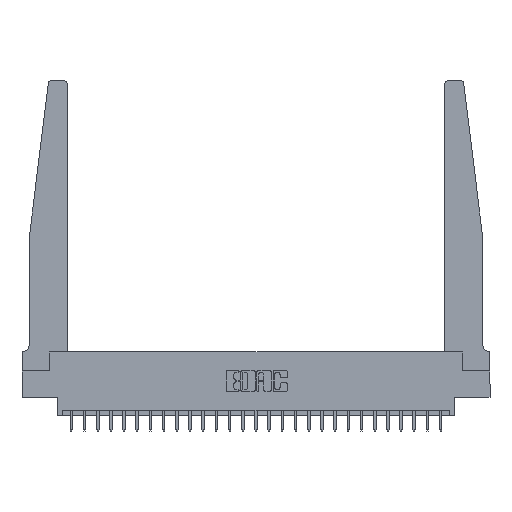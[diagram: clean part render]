
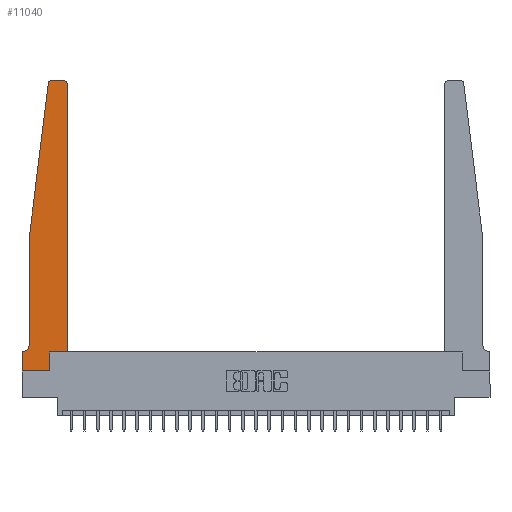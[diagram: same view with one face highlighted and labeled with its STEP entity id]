
A CAD part, top view. The second image highlights one B-rep face of the part: STEP entity #11040.
In plain terms, the highlighted planar face has unit normal (0, 0, 1).
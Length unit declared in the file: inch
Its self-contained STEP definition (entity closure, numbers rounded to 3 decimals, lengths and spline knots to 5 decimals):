
#15 = VECTOR ( 'NONE', #23621, 39.37008 ) ;
#415 = ORIENTED_EDGE ( 'NONE', *, *, #13755, .T. ) ;
#443 = CIRCLE ( 'NONE', #2517, 0.05 ) ;
#631 = CARTESIAN_POINT ( 'NONE',  ( 0.065, 0.1875, 0.37 ) ) ;
#632 = LINE ( 'NONE', #10656, #8835 ) ;
#813 = CARTESIAN_POINT ( 'NONE',  ( 0., 0., 0.37 ) ) ;
#1310 = CARTESIAN_POINT ( 'NONE',  ( 0.425, 0.18, 0.37 ) ) ;
#1545 = DIRECTION ( 'NONE',  ( 0., 0., 1. ) ) ;
#2093 = CARTESIAN_POINT ( 'NONE',  ( 0.395, 2.72, 0.37 ) ) ;
#2231 = LINE ( 'NONE', #12659, #4128 ) ;
#2368 = PLANE ( 'NONE',  #19766 ) ;
#2517 = AXIS2_PLACEMENT_3D ( 'NONE', #11095, #19156, #23111 ) ;
#2625 = ORIENTED_EDGE ( 'NONE', *, *, #9201, .T. ) ;
#3058 = VERTEX_POINT ( 'NONE', #9510 ) ;
#3242 = VECTOR ( 'NONE', #24822, 39.37008 ) ;
#3531 = LINE ( 'NONE', #3913, #18359 ) ;
#3632 = CARTESIAN_POINT ( 'NONE',  ( 0.065, 1.25, 0.37 ) ) ;
#3913 = CARTESIAN_POINT ( 'NONE',  ( 0.425, 0.18, 0.37 ) ) ;
#4128 = VECTOR ( 'NONE', #24389, 39.37008 ) ;
#5213 = ORIENTED_EDGE ( 'NONE', *, *, #22610, .T. ) ;
#5473 = VERTEX_POINT ( 'NONE', #18011 ) ;
#6308 = DIRECTION ( 'NONE',  ( 1., 0., 0. ) ) ;
#6482 = CARTESIAN_POINT ( 'NONE',  ( 0.24675, 2.72367, 0.37 ) ) ;
#6563 = LINE ( 'NONE', #631, #15560 ) ;
#6624 = EDGE_CURVE ( 'NONE', #25329, #9473, #9334, .T. ) ;
#6874 = ORIENTED_EDGE ( 'NONE', *, *, #20873, .T. ) ;
#6948 = VECTOR ( 'NONE', #25682, 39.37008 ) ;
#7537 = ORIENTED_EDGE ( 'NONE', *, *, #6624, .T. ) ;
#7592 = DIRECTION ( 'NONE',  ( 1., 0., 0. ) ) ;
#8638 = CARTESIAN_POINT ( 'NONE',  ( 0.065, 0.2375, 0.37 ) ) ;
#8674 = DIRECTION ( 'NONE',  ( -1., 0., 0. ) ) ;
#8703 = DIRECTION ( 'NONE',  ( 0., 0., 1. ) ) ;
#8835 = VECTOR ( 'NONE', #12514, 39.37008 ) ;
#9074 = VERTEX_POINT ( 'NONE', #6482 ) ;
#9201 = EDGE_CURVE ( 'NONE', #3058, #18370, #18778, .T. ) ;
#9250 = CARTESIAN_POINT ( 'NONE',  ( 0.27653, 2.75, 0.37 ) ) ;
#9334 = CIRCLE ( 'NONE', #19443, 0.03 ) ;
#9455 = CARTESIAN_POINT ( 'NONE',  ( 0.27653, 2.72, 0.37 ) ) ;
#9473 = VERTEX_POINT ( 'NONE', #9993 ) ;
#9510 = CARTESIAN_POINT ( 'NONE',  ( 0., 0., 0.37 ) ) ;
#9621 = DIRECTION ( 'NONE',  ( -1., 0., 0. ) ) ;
#9673 = EDGE_CURVE ( 'NONE', #19963, #3058, #2231, .T. ) ;
#9875 = LINE ( 'NONE', #19652, #23726 ) ;
#9993 = CARTESIAN_POINT ( 'NONE',  ( 0.395, 2.75, 0.37 ) ) ;
#10405 = DIRECTION ( 'NONE',  ( 0., 0., 1. ) ) ;
#10418 = DIRECTION ( 'NONE',  ( 1., 0., 0. ) ) ;
#10619 = CARTESIAN_POINT ( 'NONE',  ( 0.2605, 0.18, 0.37 ) ) ;
#10656 = CARTESIAN_POINT ( 'NONE',  ( 0.065, 1.25, 0.37 ) ) ;
#10702 = VERTEX_POINT ( 'NONE', #10619 ) ;
#10730 = CARTESIAN_POINT ( 'NONE',  ( 0.425, 0.18, 0.37 ) ) ;
#11040 = ADVANCED_FACE ( 'NONE', ( #20434 ), #2368, .T. ) ;
#11095 = CARTESIAN_POINT ( 'NONE',  ( 0.015, 0.2375, 0.37 ) ) ;
#11465 = EDGE_CURVE ( 'NONE', #12614, #19963, #6563, .T. ) ;
#11674 = DIRECTION ( 'NONE',  ( 0., -1., 0. ) ) ;
#11769 = EDGE_CURVE ( 'NONE', #5473, #21034, #21712, .T. ) ;
#11876 = CARTESIAN_POINT ( 'NONE',  ( 0.2605, 0.18, 0.37 ) ) ;
#12514 = DIRECTION ( 'NONE',  ( -0.122, -0.992, 0. ) ) ;
#12614 = VERTEX_POINT ( 'NONE', #19672 ) ;
#12659 = CARTESIAN_POINT ( 'NONE',  ( 0., 0., 0.37 ) ) ;
#13119 = AXIS2_PLACEMENT_3D ( 'NONE', #9455, #1545, #7592 ) ;
#13560 = LINE ( 'NONE', #1310, #6948 ) ;
#13755 = EDGE_CURVE ( 'NONE', #21034, #12614, #443, .T. ) ;
#13871 = EDGE_CURVE ( 'NONE', #18370, #10702, #25846, .T. ) ;
#14336 = ORIENTED_EDGE ( 'NONE', *, *, #16846, .T. ) ;
#15498 = CARTESIAN_POINT ( 'NONE',  ( 0.2605, 0., 0.37 ) ) ;
#15560 = VECTOR ( 'NONE', #8674, 39.37008 ) ;
#15793 = ORIENTED_EDGE ( 'NONE', *, *, #11769, .T. ) ;
#16132 = VERTEX_POINT ( 'NONE', #10730 ) ;
#16846 = EDGE_CURVE ( 'NONE', #9473, #18606, #9875, .T. ) ;
#17068 = ORIENTED_EDGE ( 'NONE', *, *, #17923, .T. ) ;
#17343 = CARTESIAN_POINT ( 'NONE',  ( 0., 0.1875, 0.37 ) ) ;
#17923 = EDGE_CURVE ( 'NONE', #16132, #25329, #13560, .T. ) ;
#18011 = CARTESIAN_POINT ( 'NONE',  ( 0.065, 1.25, 0.37 ) ) ;
#18359 = VECTOR ( 'NONE', #19642, 39.37008 ) ;
#18370 = VERTEX_POINT ( 'NONE', #15498 ) ;
#18606 = VERTEX_POINT ( 'NONE', #9250 ) ;
#18778 = LINE ( 'NONE', #813, #3242 ) ;
#19156 = DIRECTION ( 'NONE',  ( 0., 0., -1. ) ) ;
#19443 = AXIS2_PLACEMENT_3D ( 'NONE', #2093, #10405, #6308 ) ;
#19506 = ORIENTED_EDGE ( 'NONE', *, *, #9673, .T. ) ;
#19642 = DIRECTION ( 'NONE',  ( 1., 0., 0. ) ) ;
#19652 = CARTESIAN_POINT ( 'NONE',  ( 0.25, 2.75, 0.37 ) ) ;
#19672 = CARTESIAN_POINT ( 'NONE',  ( 0.015, 0.1875, 0.37 ) ) ;
#19766 = AXIS2_PLACEMENT_3D ( 'NONE', #20692, #8703, #10418 ) ;
#19963 = VERTEX_POINT ( 'NONE', #17343 ) ;
#20434 = FACE_OUTER_BOUND ( 'NONE', #23069, .T. ) ;
#20449 = EDGE_CURVE ( 'NONE', #10702, #16132, #3531, .T. ) ;
#20692 = CARTESIAN_POINT ( 'NONE',  ( 0., 0.1875, 0.37 ) ) ;
#20735 = ORIENTED_EDGE ( 'NONE', *, *, #13871, .T. ) ;
#20873 = EDGE_CURVE ( 'NONE', #18606, #9074, #21963, .T. ) ;
#21034 = VERTEX_POINT ( 'NONE', #8638 ) ;
#21712 = LINE ( 'NONE', #3632, #23178 ) ;
#21963 = CIRCLE ( 'NONE', #13119, 0.03 ) ;
#22610 = EDGE_CURVE ( 'NONE', #9074, #5473, #632, .T. ) ;
#23069 = EDGE_LOOP ( 'NONE', ( #14336, #6874, #5213, #15793, #415, #23159, #19506, #2625, #20735, #23455, #17068, #7537 ) ) ;
#23111 = DIRECTION ( 'NONE',  ( -1., 0., 0. ) ) ;
#23159 = ORIENTED_EDGE ( 'NONE', *, *, #11465, .T. ) ;
#23178 = VECTOR ( 'NONE', #11674, 39.37008 ) ;
#23455 = ORIENTED_EDGE ( 'NONE', *, *, #20449, .T. ) ;
#23621 = DIRECTION ( 'NONE',  ( 0., 1., 0. ) ) ;
#23692 = CARTESIAN_POINT ( 'NONE',  ( 0.425, 2.72, 0.37 ) ) ;
#23726 = VECTOR ( 'NONE', #9621, 39.37008 ) ;
#24389 = DIRECTION ( 'NONE',  ( 0., -1., 0. ) ) ;
#24822 = DIRECTION ( 'NONE',  ( 1., 0., 0. ) ) ;
#25329 = VERTEX_POINT ( 'NONE', #23692 ) ;
#25682 = DIRECTION ( 'NONE',  ( 0., 1., 0. ) ) ;
#25846 = LINE ( 'NONE', #11876, #15 ) ;
